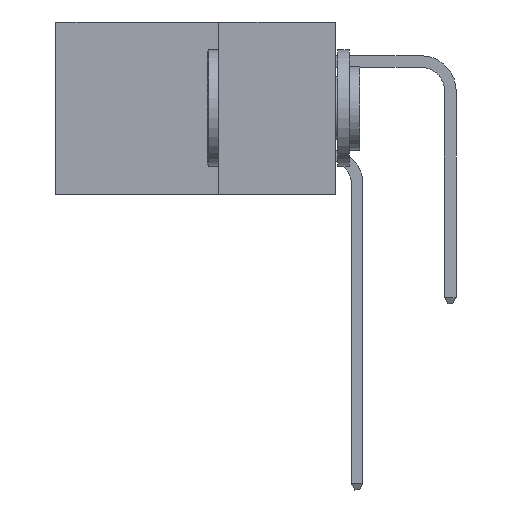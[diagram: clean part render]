
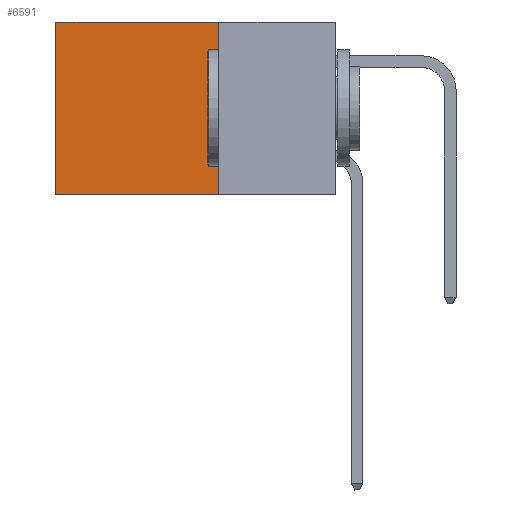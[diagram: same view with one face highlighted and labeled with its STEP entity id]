
A CAD part, left-side view. The second image highlights one B-rep face of the part: STEP entity #6591.
In plain terms, the highlighted planar face has unit normal (-1, 0, 0).
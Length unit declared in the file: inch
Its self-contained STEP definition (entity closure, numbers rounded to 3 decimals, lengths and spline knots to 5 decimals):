
#243 = VERTEX_POINT ( 'NONE', #21573 ) ;
#431 = VECTOR ( 'NONE', #19991, 39.37008 ) ;
#460 = DIRECTION ( 'NONE',  ( 1., 0., 0. ) ) ;
#1019 = ORIENTED_EDGE ( 'NONE', *, *, #5217, .T. ) ;
#1679 = DIRECTION ( 'NONE',  ( 0., 0., -1. ) ) ;
#1798 = ORIENTED_EDGE ( 'NONE', *, *, #3653, .F. ) ;
#1932 = VECTOR ( 'NONE', #20924, 39.37008 ) ;
#3653 = EDGE_CURVE ( 'NONE', #21693, #243, #12997, .T. ) ;
#4627 = CARTESIAN_POINT ( 'NONE',  ( 0.2875, 0.25, 0. ) ) ;
#5172 = AXIS2_PLACEMENT_3D ( 'NONE', #10336, #460, #14161 ) ;
#5217 = EDGE_CURVE ( 'NONE', #19336, #9801, #11152, .T. ) ;
#5681 = EDGE_CURVE ( 'NONE', #243, #9801, #5979, .T. ) ;
#5979 = LINE ( 'NONE', #19053, #1932 ) ;
#6591 = ADVANCED_FACE ( 'NONE', ( #8054 ), #17784, .F. ) ;
#6828 = CARTESIAN_POINT ( 'NONE',  ( 0.2875, 0.6, -0.37 ) ) ;
#8054 = FACE_OUTER_BOUND ( 'NONE', #9824, .T. ) ;
#9098 = EDGE_CURVE ( 'NONE', #21693, #19336, #15953, .T. ) ;
#9801 = VERTEX_POINT ( 'NONE', #6828 ) ;
#9824 = EDGE_LOOP ( 'NONE', ( #1019, #23412, #1798, #22666 ) ) ;
#10336 = CARTESIAN_POINT ( 'NONE',  ( 0.2875, 0.25, 0. ) ) ;
#11152 = LINE ( 'NONE', #22608, #15004 ) ;
#12997 = LINE ( 'NONE', #16041, #22292 ) ;
#14161 = DIRECTION ( 'NONE',  ( 0., 0., -1. ) ) ;
#15004 = VECTOR ( 'NONE', #1679, 39.37008 ) ;
#15953 = LINE ( 'NONE', #23644, #431 ) ;
#16041 = CARTESIAN_POINT ( 'NONE',  ( 0.2875, 0.25, 0. ) ) ;
#17784 = PLANE ( 'NONE',  #5172 ) ;
#17879 = DIRECTION ( 'NONE',  ( 0., 0., -1. ) ) ;
#19053 = CARTESIAN_POINT ( 'NONE',  ( 0.2875, 0.25, -0.37 ) ) ;
#19336 = VERTEX_POINT ( 'NONE', #21285 ) ;
#19991 = DIRECTION ( 'NONE',  ( 0., 1., 0. ) ) ;
#20924 = DIRECTION ( 'NONE',  ( 0., 1., 0. ) ) ;
#21285 = CARTESIAN_POINT ( 'NONE',  ( 0.2875, 0.6, 0. ) ) ;
#21573 = CARTESIAN_POINT ( 'NONE',  ( 0.2875, 0.25, -0.37 ) ) ;
#21693 = VERTEX_POINT ( 'NONE', #4627 ) ;
#22292 = VECTOR ( 'NONE', #17879, 39.37008 ) ;
#22608 = CARTESIAN_POINT ( 'NONE',  ( 0.2875, 0.6, 0. ) ) ;
#22666 = ORIENTED_EDGE ( 'NONE', *, *, #9098, .T. ) ;
#23412 = ORIENTED_EDGE ( 'NONE', *, *, #5681, .F. ) ;
#23644 = CARTESIAN_POINT ( 'NONE',  ( 0.2875, 0.25, 0. ) ) ;
